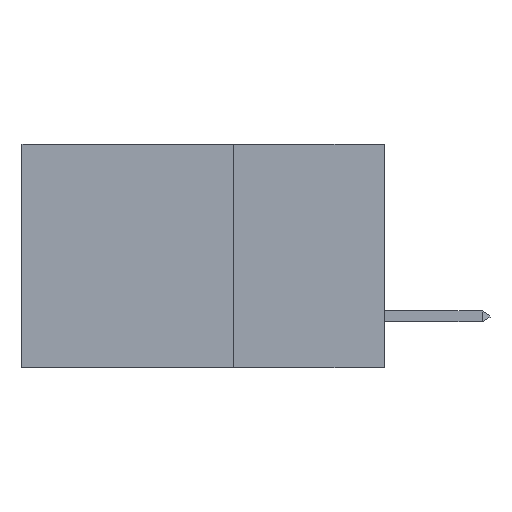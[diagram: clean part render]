
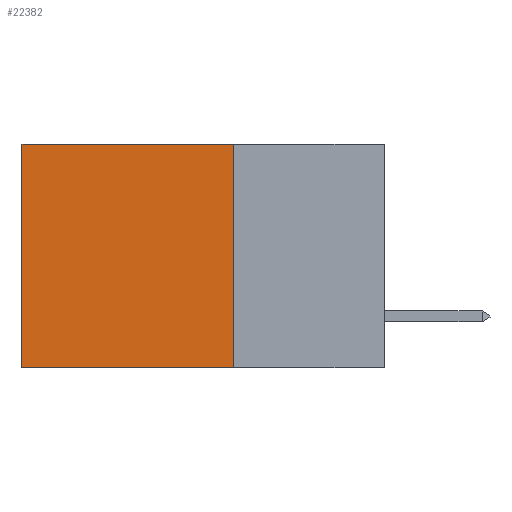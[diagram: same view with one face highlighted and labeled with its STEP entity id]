
A CAD part, left-side view. The second image highlights one B-rep face of the part: STEP entity #22382.
In plain terms, the highlighted planar face has unit normal (-1, 0, 0).
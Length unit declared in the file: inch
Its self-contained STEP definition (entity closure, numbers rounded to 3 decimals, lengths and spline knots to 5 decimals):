
#703 = VECTOR ( 'NONE', #18871, 39.37008 ) ;
#1266 = ORIENTED_EDGE ( 'NONE', *, *, #14083, .F. ) ;
#1662 = EDGE_CURVE ( 'NONE', #5413, #18777, #3132, .T. ) ;
#2422 = CARTESIAN_POINT ( 'NONE',  ( 0.2875, 0.25, 0. ) ) ;
#3132 = LINE ( 'NONE', #15254, #17185 ) ;
#4189 = DIRECTION ( 'NONE',  ( 0., 0., -1. ) ) ;
#4800 = DIRECTION ( 'NONE',  ( 0., 0., -1. ) ) ;
#5245 = EDGE_LOOP ( 'NONE', ( #5714, #1266, #22994, #7841 ) ) ;
#5413 = VERTEX_POINT ( 'NONE', #7484 ) ;
#5714 = ORIENTED_EDGE ( 'NONE', *, *, #1662, .T. ) ;
#7154 = AXIS2_PLACEMENT_3D ( 'NONE', #14073, #19503, #8604 ) ;
#7484 = CARTESIAN_POINT ( 'NONE',  ( 0.2875, 0.6, 0. ) ) ;
#7841 = ORIENTED_EDGE ( 'NONE', *, *, #22774, .T. ) ;
#8604 = DIRECTION ( 'NONE',  ( 0., 0., -1. ) ) ;
#10548 = FACE_OUTER_BOUND ( 'NONE', #5245, .T. ) ;
#11132 = VERTEX_POINT ( 'NONE', #12716 ) ;
#11217 = VERTEX_POINT ( 'NONE', #20107 ) ;
#12716 = CARTESIAN_POINT ( 'NONE',  ( 0.2875, 0.25, 0. ) ) ;
#13168 = DIRECTION ( 'NONE',  ( 0., 1., 0. ) ) ;
#13264 = CARTESIAN_POINT ( 'NONE',  ( 0.2875, 0.6, -0.37 ) ) ;
#13981 = LINE ( 'NONE', #18530, #21866 ) ;
#14073 = CARTESIAN_POINT ( 'NONE',  ( 0.2875, 0.25, 0. ) ) ;
#14083 = EDGE_CURVE ( 'NONE', #11217, #18777, #13981, .T. ) ;
#15254 = CARTESIAN_POINT ( 'NONE',  ( 0.2875, 0.6, 0. ) ) ;
#15946 = LINE ( 'NONE', #2422, #703 ) ;
#17185 = VECTOR ( 'NONE', #4189, 39.37008 ) ;
#17490 = CARTESIAN_POINT ( 'NONE',  ( 0.2875, 0.25, 0. ) ) ;
#18093 = EDGE_CURVE ( 'NONE', #11132, #11217, #18985, .T. ) ;
#18530 = CARTESIAN_POINT ( 'NONE',  ( 0.2875, 0.25, -0.37 ) ) ;
#18777 = VERTEX_POINT ( 'NONE', #13264 ) ;
#18871 = DIRECTION ( 'NONE',  ( 0., 1., 0. ) ) ;
#18985 = LINE ( 'NONE', #17490, #22619 ) ;
#19503 = DIRECTION ( 'NONE',  ( 1., 0., 0. ) ) ;
#20107 = CARTESIAN_POINT ( 'NONE',  ( 0.2875, 0.25, -0.37 ) ) ;
#21238 = PLANE ( 'NONE',  #7154 ) ;
#21866 = VECTOR ( 'NONE', #13168, 39.37008 ) ;
#22382 = ADVANCED_FACE ( 'NONE', ( #10548 ), #21238, .F. ) ;
#22619 = VECTOR ( 'NONE', #4800, 39.37008 ) ;
#22774 = EDGE_CURVE ( 'NONE', #11132, #5413, #15946, .T. ) ;
#22994 = ORIENTED_EDGE ( 'NONE', *, *, #18093, .F. ) ;
